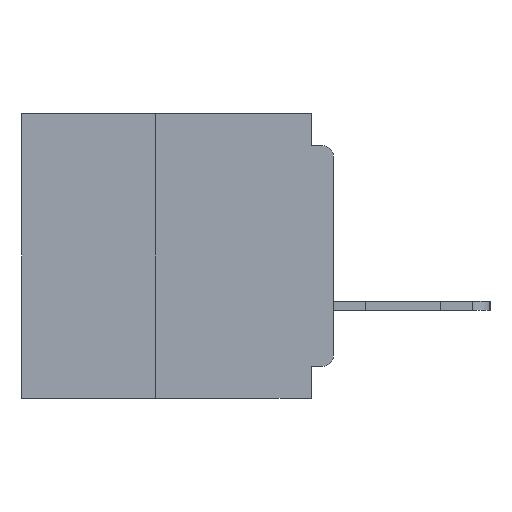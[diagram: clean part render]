
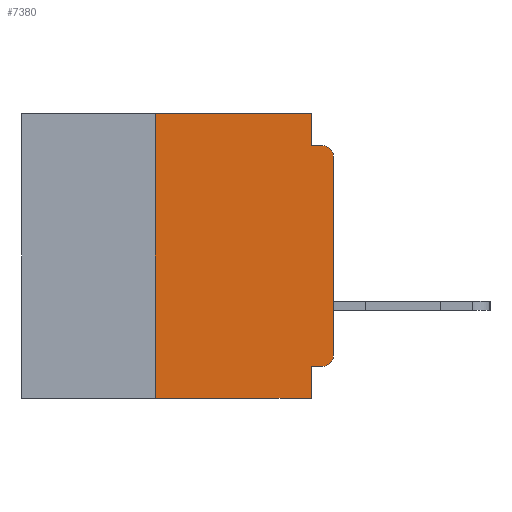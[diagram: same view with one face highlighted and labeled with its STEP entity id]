
A CAD part, left-side view. The second image highlights one B-rep face of the part: STEP entity #7380.
In plain terms, the highlighted planar face has unit normal (-1, 0, 0).
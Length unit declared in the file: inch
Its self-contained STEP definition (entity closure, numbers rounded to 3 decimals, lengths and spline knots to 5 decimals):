
#81 = CARTESIAN_POINT ( 'NONE',  ( 0., 0.437, -0.4 ) ) ;
#292 = CARTESIAN_POINT ( 'NONE',  ( 0., 0.031, -0.355 ) ) ;
#981 = ORIENTED_EDGE ( 'NONE', *, *, #21890, .F. ) ;
#1299 = AXIS2_PLACEMENT_3D ( 'NONE', #33198, #14928, #36222 ) ;
#1348 = CARTESIAN_POINT ( 'NONE',  ( 0., 0.031, 0. ) ) ;
#2067 = LINE ( 'NONE', #12465, #33547 ) ;
#2287 = EDGE_CURVE ( 'NONE', #22293, #27332, #16010, .T. ) ;
#2834 = DIRECTION ( 'NONE',  ( 0., 0., -1. ) ) ;
#3509 = LINE ( 'NONE', #7017, #33088 ) ;
#3646 = CARTESIAN_POINT ( 'NONE',  ( 0., 0., -0.34 ) ) ;
#4813 = CARTESIAN_POINT ( 'NONE',  ( 0., 0.031, -0.045 ) ) ;
#6281 = DIRECTION ( 'NONE',  ( -1., 0., 0. ) ) ;
#6394 = VERTEX_POINT ( 'NONE', #3646 ) ;
#7017 = CARTESIAN_POINT ( 'NONE',  ( 0., 0.25, -0.4 ) ) ;
#7117 = VERTEX_POINT ( 'NONE', #4813 ) ;
#7380 = ADVANCED_FACE ( 'NONE', ( #17086 ), #15160, .F. ) ;
#7651 = DIRECTION ( 'NONE',  ( 0., 0., -1. ) ) ;
#7712 = VECTOR ( 'NONE', #9276, 39.37008 ) ;
#8057 = DIRECTION ( 'NONE',  ( 0., 1., 0. ) ) ;
#8779 = CARTESIAN_POINT ( 'NONE',  ( 0., 0.015, -0.045 ) ) ;
#9119 = VERTEX_POINT ( 'NONE', #8779 ) ;
#9171 = CARTESIAN_POINT ( 'NONE',  ( 0., 0.437, 0. ) ) ;
#9276 = DIRECTION ( 'NONE',  ( 0., -1., 0. ) ) ;
#9551 = EDGE_CURVE ( 'NONE', #27915, #6394, #10277, .T. ) ;
#10105 = DIRECTION ( 'NONE',  ( 0., 0., 1. ) ) ;
#10277 = CIRCLE ( 'NONE', #33139, 0.015 ) ;
#10843 = EDGE_CURVE ( 'NONE', #6394, #11299, #2067, .T. ) ;
#11299 = VERTEX_POINT ( 'NONE', #20720 ) ;
#11790 = EDGE_LOOP ( 'NONE', ( #25144, #27799, #25620, #13929, #36977, #15089, #33845, #20494, #981, #12474 ) ) ;
#11971 = LINE ( 'NONE', #21021, #28255 ) ;
#12062 = LINE ( 'NONE', #15632, #19224 ) ;
#12245 = DIRECTION ( 'NONE',  ( 0., 0., -1. ) ) ;
#12465 = CARTESIAN_POINT ( 'NONE',  ( 0., 0., 0. ) ) ;
#12474 = ORIENTED_EDGE ( 'NONE', *, *, #9551, .T. ) ;
#13652 = EDGE_CURVE ( 'NONE', #11299, #9119, #25578, .T. ) ;
#13929 = ORIENTED_EDGE ( 'NONE', *, *, #26984, .F. ) ;
#14335 = VERTEX_POINT ( 'NONE', #15121 ) ;
#14645 = EDGE_CURVE ( 'NONE', #15568, #19338, #36824, .T. ) ;
#14928 = DIRECTION ( 'NONE',  ( -1., 0., 0. ) ) ;
#15089 = ORIENTED_EDGE ( 'NONE', *, *, #24930, .F. ) ;
#15121 = CARTESIAN_POINT ( 'NONE',  ( 0., 0.25, -0.4 ) ) ;
#15160 = PLANE ( 'NONE',  #18008 ) ;
#15503 = DIRECTION ( 'NONE',  ( 0., 0., 1. ) ) ;
#15568 = VERTEX_POINT ( 'NONE', #292 ) ;
#15632 = CARTESIAN_POINT ( 'NONE',  ( 0., 0., -0.045 ) ) ;
#16010 = LINE ( 'NONE', #22902, #16981 ) ;
#16671 = EDGE_CURVE ( 'NONE', #14335, #19338, #32068, .T. ) ;
#16981 = VECTOR ( 'NONE', #23297, 39.37008 ) ;
#17086 = FACE_OUTER_BOUND ( 'NONE', #11790, .T. ) ;
#18008 = AXIS2_PLACEMENT_3D ( 'NONE', #9171, #30560, #12245 ) ;
#19224 = VECTOR ( 'NONE', #33915, 39.37008 ) ;
#19338 = VERTEX_POINT ( 'NONE', #33582 ) ;
#20494 = ORIENTED_EDGE ( 'NONE', *, *, #14645, .F. ) ;
#20720 = CARTESIAN_POINT ( 'NONE',  ( 0., 0., -0.06 ) ) ;
#21021 = CARTESIAN_POINT ( 'NONE',  ( 0., 0.031, 0. ) ) ;
#21890 = EDGE_CURVE ( 'NONE', #27915, #15568, #27906, .T. ) ;
#22293 = VERTEX_POINT ( 'NONE', #26001 ) ;
#22902 = CARTESIAN_POINT ( 'NONE',  ( 0., 0.437, 0. ) ) ;
#23297 = DIRECTION ( 'NONE',  ( 0., -1., 0. ) ) ;
#23496 = CARTESIAN_POINT ( 'NONE',  ( 0., 0., -0.355 ) ) ;
#24601 = CARTESIAN_POINT ( 'NONE',  ( 0., 0.015, -0.34 ) ) ;
#24930 = EDGE_CURVE ( 'NONE', #14335, #22293, #3509, .T. ) ;
#25144 = ORIENTED_EDGE ( 'NONE', *, *, #10843, .T. ) ;
#25578 = CIRCLE ( 'NONE', #1299, 0.015 ) ;
#25620 = ORIENTED_EDGE ( 'NONE', *, *, #36104, .F. ) ;
#26001 = CARTESIAN_POINT ( 'NONE',  ( 0., 0.25, 0. ) ) ;
#26003 = CARTESIAN_POINT ( 'NONE',  ( 0., 0.031, -0.4 ) ) ;
#26966 = VECTOR ( 'NONE', #8057, 39.37008 ) ;
#26984 = EDGE_CURVE ( 'NONE', #27332, #7117, #11971, .T. ) ;
#27332 = VERTEX_POINT ( 'NONE', #1348 ) ;
#27674 = DIRECTION ( 'NONE',  ( 0., 0., -1. ) ) ;
#27799 = ORIENTED_EDGE ( 'NONE', *, *, #13652, .T. ) ;
#27906 = LINE ( 'NONE', #23496, #26966 ) ;
#27915 = VERTEX_POINT ( 'NONE', #29237 ) ;
#28255 = VECTOR ( 'NONE', #2834, 39.37008 ) ;
#29237 = CARTESIAN_POINT ( 'NONE',  ( 0., 0.015, -0.355 ) ) ;
#29757 = VECTOR ( 'NONE', #7651, 39.37008 ) ;
#30560 = DIRECTION ( 'NONE',  ( 1., 0., 0. ) ) ;
#32068 = LINE ( 'NONE', #81, #7712 ) ;
#33088 = VECTOR ( 'NONE', #10105, 39.37008 ) ;
#33139 = AXIS2_PLACEMENT_3D ( 'NONE', #24601, #6281, #27674 ) ;
#33198 = CARTESIAN_POINT ( 'NONE',  ( 0., 0.015, -0.06 ) ) ;
#33547 = VECTOR ( 'NONE', #15503, 39.37008 ) ;
#33582 = CARTESIAN_POINT ( 'NONE',  ( 0., 0.031, -0.4 ) ) ;
#33845 = ORIENTED_EDGE ( 'NONE', *, *, #16671, .T. ) ;
#33915 = DIRECTION ( 'NONE',  ( 0., -1., 0. ) ) ;
#36104 = EDGE_CURVE ( 'NONE', #7117, #9119, #12062, .T. ) ;
#36222 = DIRECTION ( 'NONE',  ( 0., 0., -1. ) ) ;
#36824 = LINE ( 'NONE', #26003, #29757 ) ;
#36977 = ORIENTED_EDGE ( 'NONE', *, *, #2287, .F. ) ;
